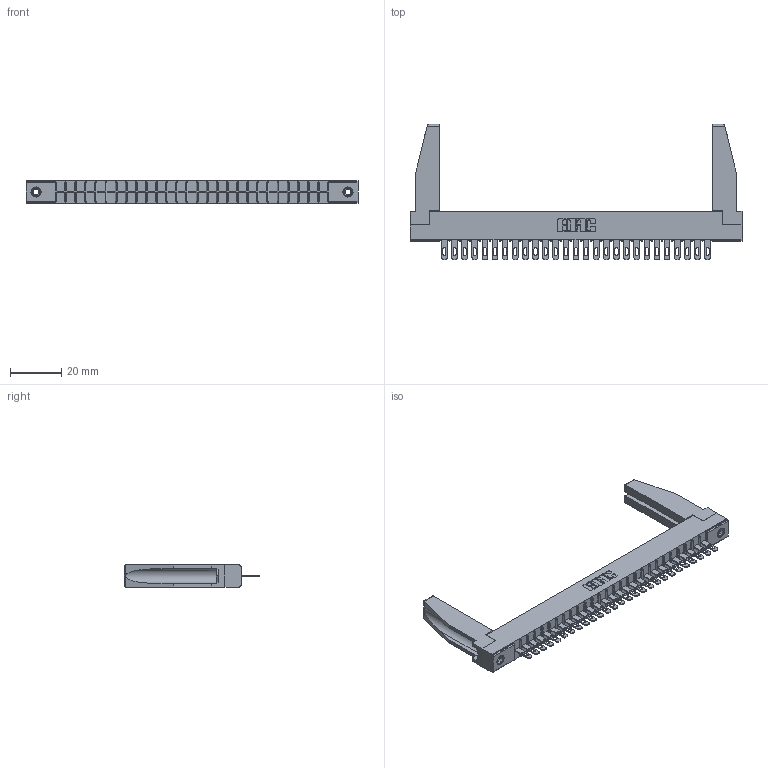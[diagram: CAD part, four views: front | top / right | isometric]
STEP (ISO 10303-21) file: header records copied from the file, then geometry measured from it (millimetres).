
FILE_DESCRIPTION (( 'STEP AP203' ), '1' );
FILE_NAME ('316-027-500-178.STEP', '2018-07-31T02:43:24', ( '' ), ( '' ), 'SwSTEP 2.0', 'SolidWorks 2016', '' );
FILE_SCHEMA (( 'CONFIG_CONTROL_DESIGN' ));
Length unit declared in the file: inch
Products named in the file (5): 306 Part_.156 Dia; 306-290-001_100; 345-250-001_345-250-001-102; 307-220-078; 316-027-500-178
Assembly tree (32 placements, depth 2):
  316-027-500-178
    306 Part_.156 Dia
    306-290-001_100  x27
    345-250-001_345-250-001-102  x2
    307-220-078  x2
Bounding box: 130 x 52.91 x 8.71 mm (x, y, z)
Volume: 12997 mm3; surface area: 17718.8 mm2
Topology: 32 solids, 32 shells, 2298 faces, 6451 edges, 4146 vertices
Faces by surface type: plane 1502, cylinder 672, sphere 108, cone 12, torus 4
Entity records: 29725 total; most frequent: CARTESIAN_POINT 4990, ORIENTED_EDGE 4904, DIRECTION 4874, EDGE_CURVE 2452, LINE 1910, VECTOR 1910, VERTEX_POINT 1556, AXIS2_PLACEMENT_3D 1482
